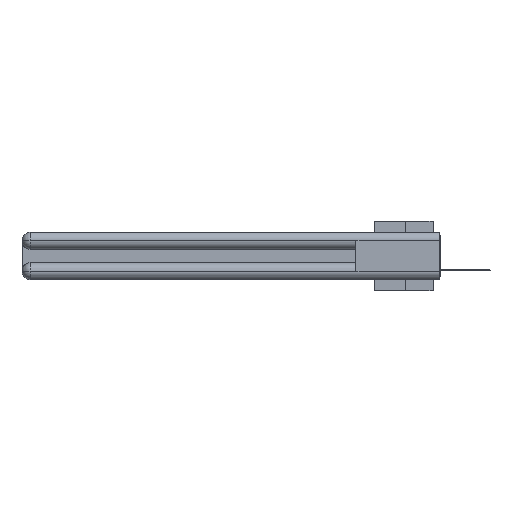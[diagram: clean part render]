
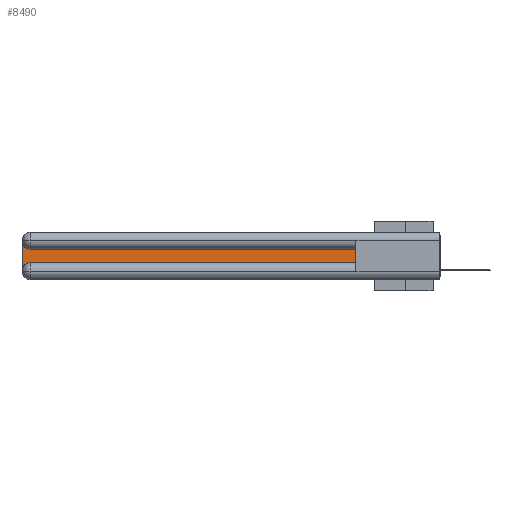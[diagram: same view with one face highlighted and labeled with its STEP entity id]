
A CAD part, left-side view. The second image highlights one B-rep face of the part: STEP entity #8490.
In plain terms, the highlighted planar face has unit normal (-1, 0, 0).
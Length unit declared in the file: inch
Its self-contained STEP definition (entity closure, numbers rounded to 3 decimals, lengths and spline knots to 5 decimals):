
#49 = EDGE_CURVE ( 'NONE', #2511, #4003, #21506, .T. ) ;
#686 = CARTESIAN_POINT ( 'NONE',  ( 0.075, 3., -0.0625 ) ) ;
#1025 = VERTEX_POINT ( 'NONE', #27796 ) ;
#1747 = CARTESIAN_POINT ( 'NONE',  ( 0.075, 2.94, -0.2175 ) ) ;
#1944 = DIRECTION ( 'NONE',  ( 1., 0., 0. ) ) ;
#2045 = FACE_OUTER_BOUND ( 'NONE', #13037, .T. ) ;
#2511 = VERTEX_POINT ( 'NONE', #30945 ) ;
#2956 = DIRECTION ( 'NONE',  ( 0., 0., -1. ) ) ;
#3062 = CARTESIAN_POINT ( 'NONE',  ( 0.075, 2.94, -0.0625 ) ) ;
#3124 = EDGE_CURVE ( 'NONE', #18663, #29218, #5924, .T. ) ;
#4003 = VERTEX_POINT ( 'NONE', #686 ) ;
#4587 = DIRECTION ( 'NONE',  ( 0., 0., -1. ) ) ;
#4828 = CARTESIAN_POINT ( 'NONE',  ( 0.075, 0.6, -0.2175 ) ) ;
#5924 = CIRCLE ( 'NONE', #14421, 0.06 ) ;
#6224 = CARTESIAN_POINT ( 'NONE',  ( 0.075, 0.6, -0.1225 ) ) ;
#6436 = EDGE_CURVE ( 'NONE', #1025, #9794, #23004, .T. ) ;
#6817 = DIRECTION ( 'NONE',  ( 1., 0., 0. ) ) ;
#7626 = ORIENTED_EDGE ( 'NONE', *, *, #23416, .T. ) ;
#7629 = CARTESIAN_POINT ( 'NONE',  ( 0.075, 2.94, -0.2775 ) ) ;
#8490 = ADVANCED_FACE ( 'NONE', ( #2045 ), #11874, .F. ) ;
#9794 = VERTEX_POINT ( 'NONE', #34032 ) ;
#10226 = LINE ( 'NONE', #11770, #23074 ) ;
#10892 = LINE ( 'NONE', #6224, #20468 ) ;
#11355 = VECTOR ( 'NONE', #12716, 39.37008 ) ;
#11770 = CARTESIAN_POINT ( 'NONE',  ( 0.075, 3., -0.2175 ) ) ;
#11874 = PLANE ( 'NONE',  #24519 ) ;
#12716 = DIRECTION ( 'NONE',  ( 0., 0., 1. ) ) ;
#13037 = EDGE_LOOP ( 'NONE', ( #21465, #15584, #13770, #28806, #7626, #14969 ) ) ;
#13301 = AXIS2_PLACEMENT_3D ( 'NONE', #3062, #18840, #2956 ) ;
#13770 = ORIENTED_EDGE ( 'NONE', *, *, #21487, .T. ) ;
#14421 = AXIS2_PLACEMENT_3D ( 'NONE', #7629, #1944, #4587 ) ;
#14969 = ORIENTED_EDGE ( 'NONE', *, *, #6436, .T. ) ;
#15584 = ORIENTED_EDGE ( 'NONE', *, *, #49, .T. ) ;
#17111 = DIRECTION ( 'NONE',  ( 0., 0., -1. ) ) ;
#18663 = VERTEX_POINT ( 'NONE', #29670 ) ;
#18840 = DIRECTION ( 'NONE',  ( 1., 0., 0. ) ) ;
#20468 = VECTOR ( 'NONE', #27281, 39.37008 ) ;
#21292 = DIRECTION ( 'NONE',  ( 0., -1., 0. ) ) ;
#21465 = ORIENTED_EDGE ( 'NONE', *, *, #23847, .T. ) ;
#21487 = EDGE_CURVE ( 'NONE', #4003, #18663, #10226, .T. ) ;
#21506 = CIRCLE ( 'NONE', #13301, 0.06 ) ;
#23004 = LINE ( 'NONE', #4828, #11355 ) ;
#23074 = VECTOR ( 'NONE', #17111, 39.37008 ) ;
#23416 = EDGE_CURVE ( 'NONE', #29218, #1025, #33762, .T. ) ;
#23847 = EDGE_CURVE ( 'NONE', #9794, #2511, #10892, .T. ) ;
#24519 = AXIS2_PLACEMENT_3D ( 'NONE', #33186, #6817, #25348 ) ;
#25064 = VECTOR ( 'NONE', #21292, 39.37008 ) ;
#25348 = DIRECTION ( 'NONE',  ( 0., 0., -1. ) ) ;
#27281 = DIRECTION ( 'NONE',  ( 0., 1., 0. ) ) ;
#27796 = CARTESIAN_POINT ( 'NONE',  ( 0.075, 0.6, -0.2175 ) ) ;
#28806 = ORIENTED_EDGE ( 'NONE', *, *, #3124, .T. ) ;
#29218 = VERTEX_POINT ( 'NONE', #1747 ) ;
#29670 = CARTESIAN_POINT ( 'NONE',  ( 0.075, 3., -0.2775 ) ) ;
#30945 = CARTESIAN_POINT ( 'NONE',  ( 0.075, 2.94, -0.1225 ) ) ;
#32179 = CARTESIAN_POINT ( 'NONE',  ( 0.075, 0.6, -0.2175 ) ) ;
#33186 = CARTESIAN_POINT ( 'NONE',  ( 0.075, 3., -0.1225 ) ) ;
#33762 = LINE ( 'NONE', #32179, #25064 ) ;
#34032 = CARTESIAN_POINT ( 'NONE',  ( 0.075, 0.6, -0.1225 ) ) ;
